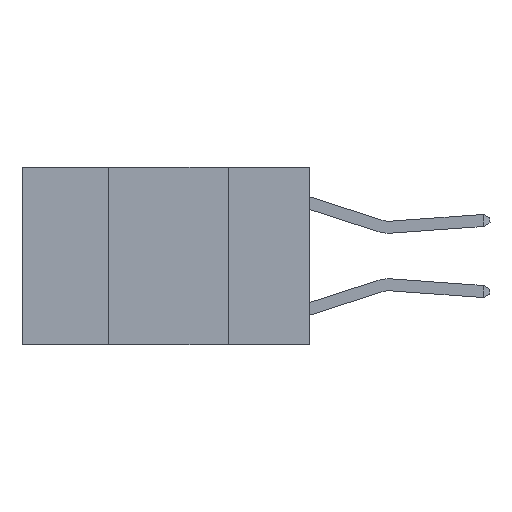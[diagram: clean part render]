
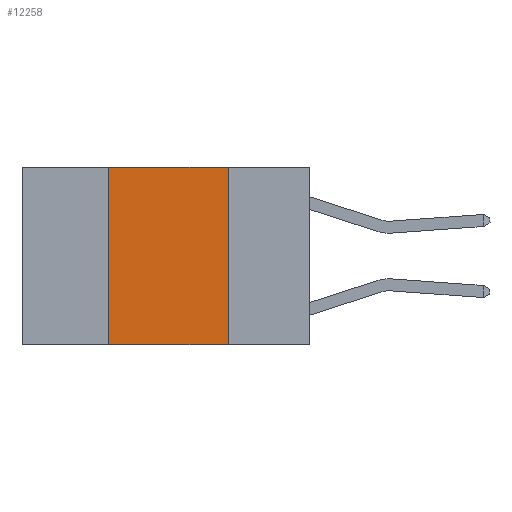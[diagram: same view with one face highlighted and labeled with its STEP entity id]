
A CAD part, left-side view. The second image highlights one B-rep face of the part: STEP entity #12258.
In plain terms, the highlighted planar face has unit normal (-1, 0, 0).
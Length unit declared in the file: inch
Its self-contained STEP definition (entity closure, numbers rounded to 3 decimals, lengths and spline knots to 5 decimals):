
#86 = ORIENTED_EDGE ( 'NONE', *, *, #26576, .T. ) ;
#900 = DIRECTION ( 'NONE',  ( 0., -1., 0. ) ) ;
#2411 = VECTOR ( 'NONE', #21153, 39.37008 ) ;
#2419 = VERTEX_POINT ( 'NONE', #23885 ) ;
#3215 = CARTESIAN_POINT ( 'NONE',  ( 0., 0.6, -0.37 ) ) ;
#3906 = VECTOR ( 'NONE', #28395, 39.37008 ) ;
#5281 = CARTESIAN_POINT ( 'NONE',  ( 0., 0.6, 0. ) ) ;
#6317 = EDGE_LOOP ( 'NONE', ( #10102, #10844, #16873, #86 ) ) ;
#6477 = CARTESIAN_POINT ( 'NONE',  ( 0., 0.17, 0. ) ) ;
#7556 = CARTESIAN_POINT ( 'NONE',  ( 0., 0.42, 0. ) ) ;
#8469 = LINE ( 'NONE', #5281, #2411 ) ;
#8758 = DIRECTION ( 'NONE',  ( 0., 0., -1. ) ) ;
#9995 = LINE ( 'NONE', #17135, #3906 ) ;
#10102 = ORIENTED_EDGE ( 'NONE', *, *, #26095, .F. ) ;
#10192 = CARTESIAN_POINT ( 'NONE',  ( 0., 0.6, 0. ) ) ;
#10844 = ORIENTED_EDGE ( 'NONE', *, *, #20773, .F. ) ;
#10976 = LINE ( 'NONE', #3215, #17001 ) ;
#12258 = ADVANCED_FACE ( 'NONE', ( #28568 ), #12533, .F. ) ;
#12533 = PLANE ( 'NONE',  #24875 ) ;
#14667 = VERTEX_POINT ( 'NONE', #7556 ) ;
#14786 = DIRECTION ( 'NONE',  ( 0., 0., -1. ) ) ;
#16312 = VECTOR ( 'NONE', #8758, 39.37008 ) ;
#16873 = ORIENTED_EDGE ( 'NONE', *, *, #18672, .F. ) ;
#17001 = VECTOR ( 'NONE', #900, 39.37008 ) ;
#17135 = CARTESIAN_POINT ( 'NONE',  ( 0., 0.42, 0. ) ) ;
#17738 = LINE ( 'NONE', #6477, #16312 ) ;
#18156 = CARTESIAN_POINT ( 'NONE',  ( 0., 0.17, -0.37 ) ) ;
#18672 = EDGE_CURVE ( 'NONE', #22335, #14667, #9995, .T. ) ;
#20773 = EDGE_CURVE ( 'NONE', #14667, #2419, #8469, .T. ) ;
#21153 = DIRECTION ( 'NONE',  ( 0., -1., 0. ) ) ;
#22268 = CARTESIAN_POINT ( 'NONE',  ( 0., 0.42, -0.37 ) ) ;
#22335 = VERTEX_POINT ( 'NONE', #22268 ) ;
#23308 = VERTEX_POINT ( 'NONE', #18156 ) ;
#23885 = CARTESIAN_POINT ( 'NONE',  ( 0., 0.17, 0. ) ) ;
#24875 = AXIS2_PLACEMENT_3D ( 'NONE', #10192, #28229, #14786 ) ;
#26095 = EDGE_CURVE ( 'NONE', #2419, #23308, #17738, .T. ) ;
#26576 = EDGE_CURVE ( 'NONE', #22335, #23308, #10976, .T. ) ;
#28229 = DIRECTION ( 'NONE',  ( 1., 0., 0. ) ) ;
#28395 = DIRECTION ( 'NONE',  ( 0., 0., 1. ) ) ;
#28568 = FACE_OUTER_BOUND ( 'NONE', #6317, .T. ) ;
